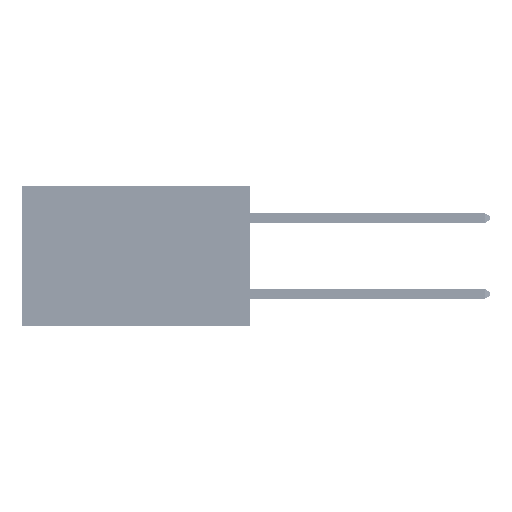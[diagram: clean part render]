
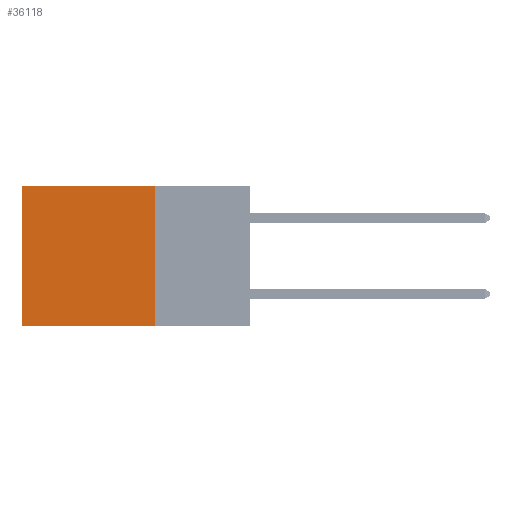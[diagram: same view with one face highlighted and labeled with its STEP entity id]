
A CAD part, left-side view. The second image highlights one B-rep face of the part: STEP entity #36118.
In plain terms, the highlighted planar face has unit normal (-1, 0, 0).
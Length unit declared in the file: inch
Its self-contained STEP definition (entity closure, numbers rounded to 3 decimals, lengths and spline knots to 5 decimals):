
#5856 = ORIENTED_EDGE ( 'NONE', *, *, #7002, .F. ) ;
#6258 = ORIENTED_EDGE ( 'NONE', *, *, #33280, .F. ) ;
#7002 = EDGE_CURVE ( 'NONE', #43149, #9880, #16617, .T. ) ;
#7608 = EDGE_LOOP ( 'NONE', ( #32908, #5856, #6258, #42687 ) ) ;
#9170 = AXIS2_PLACEMENT_3D ( 'NONE', #49262, #13546, #41673 ) ;
#9880 = VERTEX_POINT ( 'NONE', #39118 ) ;
#12370 = CARTESIAN_POINT ( 'NONE',  ( 0.2875, 0.25, 0. ) ) ;
#13546 = DIRECTION ( 'NONE',  ( 1., 0., 0. ) ) ;
#13737 = VECTOR ( 'NONE', #16496, 39.37008 ) ;
#16496 = DIRECTION ( 'NONE',  ( 0., 0., -1. ) ) ;
#16617 = LINE ( 'NONE', #43521, #35465 ) ;
#17330 = LINE ( 'NONE', #48368, #26815 ) ;
#18211 = CARTESIAN_POINT ( 'NONE',  ( 0.2875, 0.6, 0. ) ) ;
#18414 = LINE ( 'NONE', #18211, #38435 ) ;
#20679 = DIRECTION ( 'NONE',  ( 0., 1., 0. ) ) ;
#22293 = DIRECTION ( 'NONE',  ( 0., 0., -1. ) ) ;
#23352 = EDGE_CURVE ( 'NONE', #49791, #9880, #18414, .T. ) ;
#24890 = CARTESIAN_POINT ( 'NONE',  ( 0.2875, 0.25, -0.37 ) ) ;
#26750 = CARTESIAN_POINT ( 'NONE',  ( 0.2875, 0.6, 0. ) ) ;
#26815 = VECTOR ( 'NONE', #20679, 39.37008 ) ;
#28340 = FACE_OUTER_BOUND ( 'NONE', #7608, .T. ) ;
#32908 = ORIENTED_EDGE ( 'NONE', *, *, #23352, .T. ) ;
#33280 = EDGE_CURVE ( 'NONE', #36365, #43149, #45739, .T. ) ;
#33646 = PLANE ( 'NONE',  #9170 ) ;
#35465 = VECTOR ( 'NONE', #47488, 39.37008 ) ;
#36118 = ADVANCED_FACE ( 'NONE', ( #28340 ), #33646, .F. ) ;
#36365 = VERTEX_POINT ( 'NONE', #38684 ) ;
#38435 = VECTOR ( 'NONE', #22293, 39.37008 ) ;
#38684 = CARTESIAN_POINT ( 'NONE',  ( 0.2875, 0.25, 0. ) ) ;
#39118 = CARTESIAN_POINT ( 'NONE',  ( 0.2875, 0.6, -0.37 ) ) ;
#39504 = EDGE_CURVE ( 'NONE', #36365, #49791, #17330, .T. ) ;
#41673 = DIRECTION ( 'NONE',  ( 0., 0., -1. ) ) ;
#42687 = ORIENTED_EDGE ( 'NONE', *, *, #39504, .T. ) ;
#43149 = VERTEX_POINT ( 'NONE', #24890 ) ;
#43521 = CARTESIAN_POINT ( 'NONE',  ( 0.2875, 0.25, -0.37 ) ) ;
#45739 = LINE ( 'NONE', #12370, #13737 ) ;
#47488 = DIRECTION ( 'NONE',  ( 0., 1., 0. ) ) ;
#48368 = CARTESIAN_POINT ( 'NONE',  ( 0.2875, 0.25, 0. ) ) ;
#49262 = CARTESIAN_POINT ( 'NONE',  ( 0.2875, 0.25, 0. ) ) ;
#49791 = VERTEX_POINT ( 'NONE', #26750 ) ;
